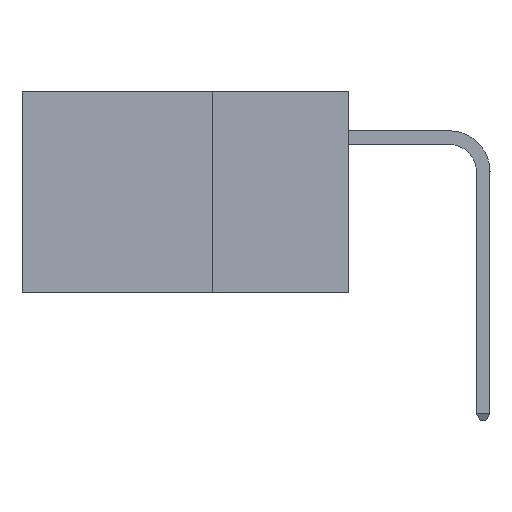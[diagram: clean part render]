
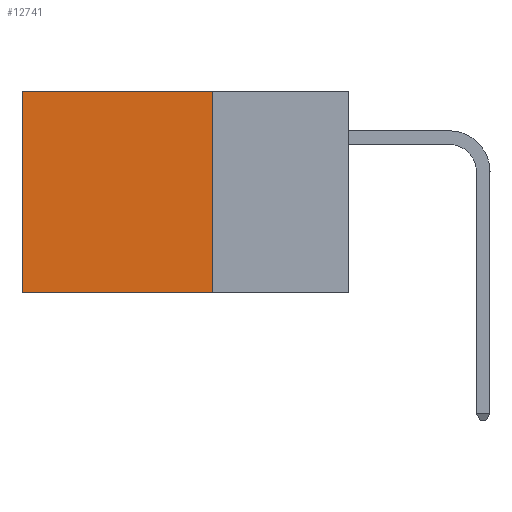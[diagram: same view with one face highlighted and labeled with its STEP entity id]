
A CAD part, left-side view. The second image highlights one B-rep face of the part: STEP entity #12741.
In plain terms, the highlighted planar face has unit normal (-1, 0, 0).
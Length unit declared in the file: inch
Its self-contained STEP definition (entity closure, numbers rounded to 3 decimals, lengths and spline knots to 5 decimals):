
#1055 = DIRECTION ( 'NONE',  ( 0., 1., 0. ) ) ;
#1541 = CARTESIAN_POINT ( 'NONE',  ( 0.2875, 0.25, 0. ) ) ;
#2162 = CARTESIAN_POINT ( 'NONE',  ( 0.2875, 0.25, -0.37 ) ) ;
#2784 = VECTOR ( 'NONE', #31820, 39.37008 ) ;
#3619 = CARTESIAN_POINT ( 'NONE',  ( 0.2875, 0.6, 0. ) ) ;
#5366 = DIRECTION ( 'NONE',  ( 0., 1., 0. ) ) ;
#6776 = LINE ( 'NONE', #2162, #22802 ) ;
#7624 = DIRECTION ( 'NONE',  ( 0., 0., -1. ) ) ;
#9160 = ORIENTED_EDGE ( 'NONE', *, *, #37793, .F. ) ;
#9375 = CARTESIAN_POINT ( 'NONE',  ( 0.2875, 0.25, 0. ) ) ;
#9593 = VERTEX_POINT ( 'NONE', #11597 ) ;
#9978 = EDGE_CURVE ( 'NONE', #10110, #9593, #24254, .T. ) ;
#10110 = VERTEX_POINT ( 'NONE', #3619 ) ;
#10349 = EDGE_LOOP ( 'NONE', ( #24938, #12388, #9160, #12935 ) ) ;
#10579 = EDGE_CURVE ( 'NONE', #17031, #10110, #39759, .T. ) ;
#11588 = CARTESIAN_POINT ( 'NONE',  ( 0.2875, 0.25, 0. ) ) ;
#11597 = CARTESIAN_POINT ( 'NONE',  ( 0.2875, 0.6, -0.37 ) ) ;
#12388 = ORIENTED_EDGE ( 'NONE', *, *, #24880, .F. ) ;
#12741 = ADVANCED_FACE ( 'NONE', ( #25814 ), #20091, .F. ) ;
#12861 = CARTESIAN_POINT ( 'NONE',  ( 0.2875, 0.25, -0.37 ) ) ;
#12935 = ORIENTED_EDGE ( 'NONE', *, *, #10579, .T. ) ;
#13805 = DIRECTION ( 'NONE',  ( 1., 0., 0. ) ) ;
#13807 = LINE ( 'NONE', #9375, #2784 ) ;
#17031 = VERTEX_POINT ( 'NONE', #11588 ) ;
#18211 = VECTOR ( 'NONE', #1055, 39.37008 ) ;
#18506 = AXIS2_PLACEMENT_3D ( 'NONE', #23576, #13805, #7624 ) ;
#20091 = PLANE ( 'NONE',  #18506 ) ;
#22802 = VECTOR ( 'NONE', #5366, 39.37008 ) ;
#23576 = CARTESIAN_POINT ( 'NONE',  ( 0.2875, 0.25, 0. ) ) ;
#24254 = LINE ( 'NONE', #29728, #28758 ) ;
#24880 = EDGE_CURVE ( 'NONE', #40099, #9593, #6776, .T. ) ;
#24938 = ORIENTED_EDGE ( 'NONE', *, *, #9978, .T. ) ;
#25814 = FACE_OUTER_BOUND ( 'NONE', #10349, .T. ) ;
#28758 = VECTOR ( 'NONE', #32996, 39.37008 ) ;
#29728 = CARTESIAN_POINT ( 'NONE',  ( 0.2875, 0.6, 0. ) ) ;
#31820 = DIRECTION ( 'NONE',  ( 0., 0., -1. ) ) ;
#32996 = DIRECTION ( 'NONE',  ( 0., 0., -1. ) ) ;
#37793 = EDGE_CURVE ( 'NONE', #17031, #40099, #13807, .T. ) ;
#39759 = LINE ( 'NONE', #1541, #18211 ) ;
#40099 = VERTEX_POINT ( 'NONE', #12861 ) ;
